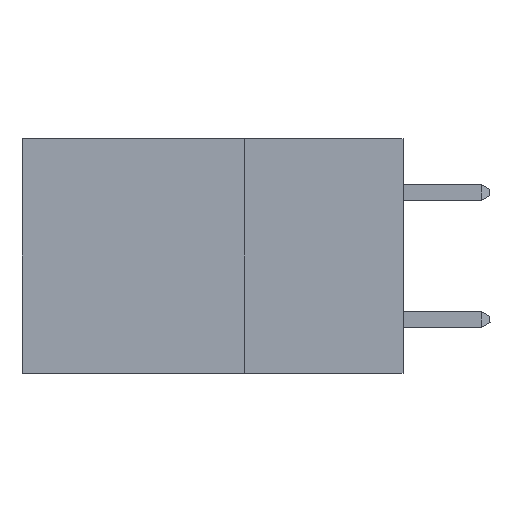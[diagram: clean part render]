
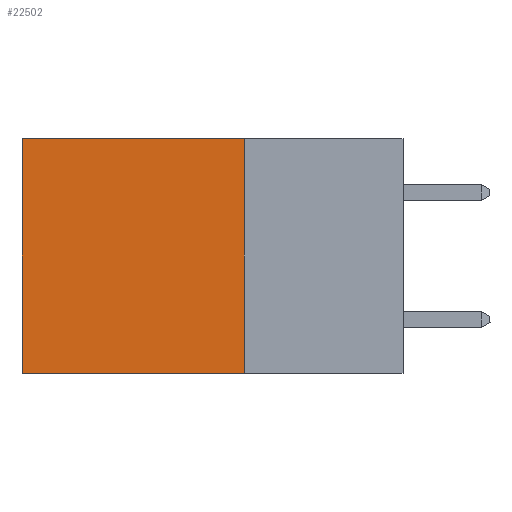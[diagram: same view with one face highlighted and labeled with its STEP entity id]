
A CAD part, left-side view. The second image highlights one B-rep face of the part: STEP entity #22502.
In plain terms, the highlighted planar face has unit normal (-1, 0, 0).
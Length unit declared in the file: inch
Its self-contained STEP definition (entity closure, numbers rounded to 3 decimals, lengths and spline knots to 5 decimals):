
#365 = EDGE_CURVE ( 'NONE', #14063, #16191, #20899, .T. ) ;
#1183 = CARTESIAN_POINT ( 'NONE',  ( 0.2875, 0.25, -0.37 ) ) ;
#1193 = VERTEX_POINT ( 'NONE', #16450 ) ;
#2791 = CARTESIAN_POINT ( 'NONE',  ( 0.2875, 0.6, 0. ) ) ;
#4909 = PLANE ( 'NONE',  #10660 ) ;
#5187 = EDGE_LOOP ( 'NONE', ( #15674, #24063, #5657, #12186 ) ) ;
#5525 = LINE ( 'NONE', #28726, #10117 ) ;
#5657 = ORIENTED_EDGE ( 'NONE', *, *, #21618, .F. ) ;
#6976 = FACE_OUTER_BOUND ( 'NONE', #5187, .T. ) ;
#7071 = DIRECTION ( 'NONE',  ( 1., 0., 0. ) ) ;
#7233 = CARTESIAN_POINT ( 'NONE',  ( 0.2875, 0.25, 0. ) ) ;
#8612 = LINE ( 'NONE', #2791, #15658 ) ;
#8747 = CARTESIAN_POINT ( 'NONE',  ( 0.2875, 0.6, 0. ) ) ;
#9498 = DIRECTION ( 'NONE',  ( 0., 1., 0. ) ) ;
#10117 = VECTOR ( 'NONE', #17127, 39.37008 ) ;
#10660 = AXIS2_PLACEMENT_3D ( 'NONE', #13781, #7071, #18045 ) ;
#12186 = ORIENTED_EDGE ( 'NONE', *, *, #365, .T. ) ;
#12519 = DIRECTION ( 'NONE',  ( 0., 0., -1. ) ) ;
#13046 = VECTOR ( 'NONE', #12519, 39.37008 ) ;
#13265 = EDGE_CURVE ( 'NONE', #18580, #1193, #5525, .T. ) ;
#13781 = CARTESIAN_POINT ( 'NONE',  ( 0.2875, 0.25, 0. ) ) ;
#14063 = VERTEX_POINT ( 'NONE', #15318 ) ;
#15318 = CARTESIAN_POINT ( 'NONE',  ( 0.2875, 0.25, 0. ) ) ;
#15408 = CARTESIAN_POINT ( 'NONE',  ( 0.2875, 0.25, 0. ) ) ;
#15537 = LINE ( 'NONE', #15408, #13046 ) ;
#15658 = VECTOR ( 'NONE', #16250, 39.37008 ) ;
#15674 = ORIENTED_EDGE ( 'NONE', *, *, #27237, .T. ) ;
#16191 = VERTEX_POINT ( 'NONE', #8747 ) ;
#16250 = DIRECTION ( 'NONE',  ( 0., 0., -1. ) ) ;
#16450 = CARTESIAN_POINT ( 'NONE',  ( 0.2875, 0.6, -0.37 ) ) ;
#17127 = DIRECTION ( 'NONE',  ( 0., 1., 0. ) ) ;
#18045 = DIRECTION ( 'NONE',  ( 0., 0., -1. ) ) ;
#18580 = VERTEX_POINT ( 'NONE', #1183 ) ;
#19152 = VECTOR ( 'NONE', #9498, 39.37008 ) ;
#20899 = LINE ( 'NONE', #7233, #19152 ) ;
#21618 = EDGE_CURVE ( 'NONE', #14063, #18580, #15537, .T. ) ;
#22502 = ADVANCED_FACE ( 'NONE', ( #6976 ), #4909, .F. ) ;
#24063 = ORIENTED_EDGE ( 'NONE', *, *, #13265, .F. ) ;
#27237 = EDGE_CURVE ( 'NONE', #16191, #1193, #8612, .T. ) ;
#28726 = CARTESIAN_POINT ( 'NONE',  ( 0.2875, 0.25, -0.37 ) ) ;
